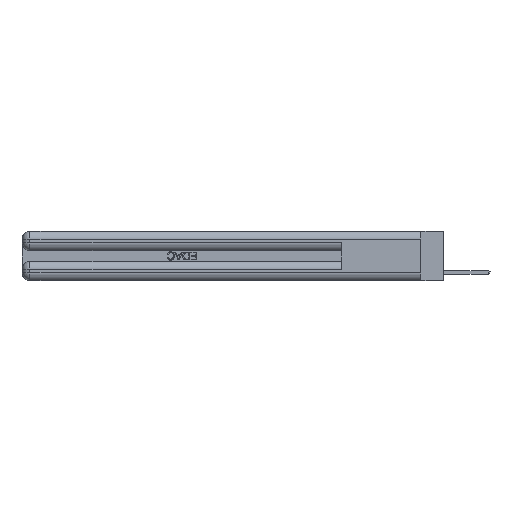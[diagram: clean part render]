
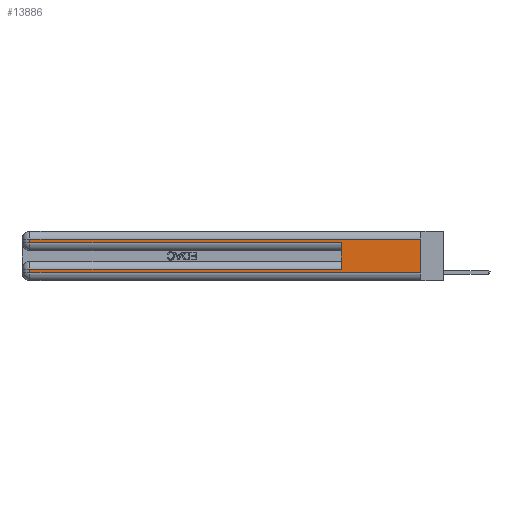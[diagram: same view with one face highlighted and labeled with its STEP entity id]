
A CAD part, left-side view. The second image highlights one B-rep face of the part: STEP entity #13886.
In plain terms, the highlighted planar face has unit normal (-1, 0, 0).
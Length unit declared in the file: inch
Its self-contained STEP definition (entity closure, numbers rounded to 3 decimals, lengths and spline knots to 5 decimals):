
#511 = DIRECTION ( 'NONE',  ( 0., -1., 0. ) ) ;
#921 = CARTESIAN_POINT ( 'NONE',  ( 0., 0.6, 0.145 ) ) ;
#1033 = LINE ( 'NONE', #26032, #8542 ) ;
#1070 = ORIENTED_EDGE ( 'NONE', *, *, #14049, .F. ) ;
#1638 = ORIENTED_EDGE ( 'NONE', *, *, #13676, .T. ) ;
#1714 = VERTEX_POINT ( 'NONE', #15985 ) ;
#1994 = VECTOR ( 'NONE', #27540, 39.37008 ) ;
#3185 = CARTESIAN_POINT ( 'NONE',  ( 0., 0., 0.37 ) ) ;
#3408 = EDGE_CURVE ( 'NONE', #15310, #18430, #25906, .T. ) ;
#3459 = ORIENTED_EDGE ( 'NONE', *, *, #13523, .T. ) ;
#3888 = EDGE_CURVE ( 'NONE', #15065, #18430, #6945, .T. ) ;
#4249 = ORIENTED_EDGE ( 'NONE', *, *, #17287, .T. ) ;
#4432 = LINE ( 'NONE', #27193, #20410 ) ;
#4941 = VECTOR ( 'NONE', #511, 39.37008 ) ;
#6811 = CARTESIAN_POINT ( 'NONE',  ( 0., 2.94, 0.37 ) ) ;
#6945 = LINE ( 'NONE', #25355, #4941 ) ;
#7158 = AXIS2_PLACEMENT_3D ( 'NONE', #3185, #21920, #25833 ) ;
#7278 = LINE ( 'NONE', #6811, #22313 ) ;
#8207 = DIRECTION ( 'NONE',  ( 0., 0., -1. ) ) ;
#8542 = VECTOR ( 'NONE', #21564, 39.37008 ) ;
#10013 = CARTESIAN_POINT ( 'NONE',  ( 0., 2.94, 0.285 ) ) ;
#11499 = CARTESIAN_POINT ( 'NONE',  ( 0., 0., 0.085 ) ) ;
#11873 = DIRECTION ( 'NONE',  ( 0., 0., -1. ) ) ;
#12138 = LINE ( 'NONE', #921, #23832 ) ;
#13499 = DIRECTION ( 'NONE',  ( 0., 1., 0. ) ) ;
#13523 = EDGE_CURVE ( 'NONE', #14093, #1714, #1033, .T. ) ;
#13647 = VERTEX_POINT ( 'NONE', #22677 ) ;
#13676 = EDGE_CURVE ( 'NONE', #15310, #25092, #4432, .T. ) ;
#13886 = ADVANCED_FACE ( 'NONE', ( #14660 ), #17352, .F. ) ;
#14049 = EDGE_CURVE ( 'NONE', #28573, #1714, #12138, .T. ) ;
#14093 = VERTEX_POINT ( 'NONE', #10013 ) ;
#14612 = DIRECTION ( 'NONE',  ( 0., 0., -1. ) ) ;
#14660 = FACE_OUTER_BOUND ( 'NONE', #18867, .T. ) ;
#15065 = VERTEX_POINT ( 'NONE', #26431 ) ;
#15310 = VERTEX_POINT ( 'NONE', #23544 ) ;
#15843 = VECTOR ( 'NONE', #14612, 39.37008 ) ;
#15985 = CARTESIAN_POINT ( 'NONE',  ( 0., 0.6, 0.285 ) ) ;
#16420 = LINE ( 'NONE', #11499, #1994 ) ;
#16954 = LINE ( 'NONE', #17269, #17076 ) ;
#17076 = VECTOR ( 'NONE', #8207, 39.37008 ) ;
#17269 = CARTESIAN_POINT ( 'NONE',  ( 0., 2.94, 0.37 ) ) ;
#17287 = EDGE_CURVE ( 'NONE', #13647, #15065, #16954, .T. ) ;
#17315 = ORIENTED_EDGE ( 'NONE', *, *, #22109, .T. ) ;
#17352 = PLANE ( 'NONE',  #7158 ) ;
#18430 = VERTEX_POINT ( 'NONE', #24073 ) ;
#18840 = CARTESIAN_POINT ( 'NONE',  ( 0., 2.94, 0.31 ) ) ;
#18867 = EDGE_LOOP ( 'NONE', ( #19033, #1638, #17315, #3459, #1070, #26084, #4249, #21123 ) ) ;
#19033 = ORIENTED_EDGE ( 'NONE', *, *, #3408, .F. ) ;
#20410 = VECTOR ( 'NONE', #13499, 39.37008 ) ;
#21123 = ORIENTED_EDGE ( 'NONE', *, *, #3888, .T. ) ;
#21564 = DIRECTION ( 'NONE',  ( 0., -1., 0. ) ) ;
#21920 = DIRECTION ( 'NONE',  ( 1., 0., 0. ) ) ;
#22109 = EDGE_CURVE ( 'NONE', #25092, #14093, #7278, .T. ) ;
#22313 = VECTOR ( 'NONE', #11873, 39.37008 ) ;
#22677 = CARTESIAN_POINT ( 'NONE',  ( 0., 2.94, 0.085 ) ) ;
#23485 = CARTESIAN_POINT ( 'NONE',  ( 0., 0.6, 0.085 ) ) ;
#23544 = CARTESIAN_POINT ( 'NONE',  ( 0., 0., 0.31 ) ) ;
#23832 = VECTOR ( 'NONE', #26243, 39.37008 ) ;
#24073 = CARTESIAN_POINT ( 'NONE',  ( 0., 0., 0.06 ) ) ;
#25092 = VERTEX_POINT ( 'NONE', #18840 ) ;
#25355 = CARTESIAN_POINT ( 'NONE',  ( 0., 0., 0.06 ) ) ;
#25558 = EDGE_CURVE ( 'NONE', #28573, #13647, #16420, .T. ) ;
#25833 = DIRECTION ( 'NONE',  ( 0., 0., -1. ) ) ;
#25906 = LINE ( 'NONE', #28704, #15843 ) ;
#26032 = CARTESIAN_POINT ( 'NONE',  ( 0., 0., 0.285 ) ) ;
#26084 = ORIENTED_EDGE ( 'NONE', *, *, #25558, .T. ) ;
#26243 = DIRECTION ( 'NONE',  ( 0., 0., 1. ) ) ;
#26431 = CARTESIAN_POINT ( 'NONE',  ( 0., 2.94, 0.06 ) ) ;
#27193 = CARTESIAN_POINT ( 'NONE',  ( 0., 0., 0.31 ) ) ;
#27540 = DIRECTION ( 'NONE',  ( 0., 1., 0. ) ) ;
#28573 = VERTEX_POINT ( 'NONE', #23485 ) ;
#28704 = CARTESIAN_POINT ( 'NONE',  ( 0., 0., 0.37 ) ) ;
